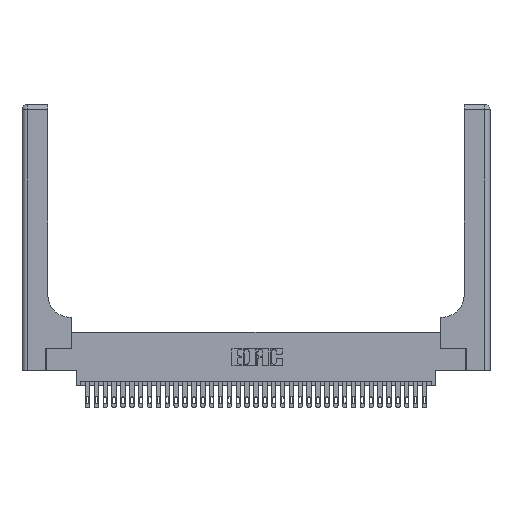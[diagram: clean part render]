
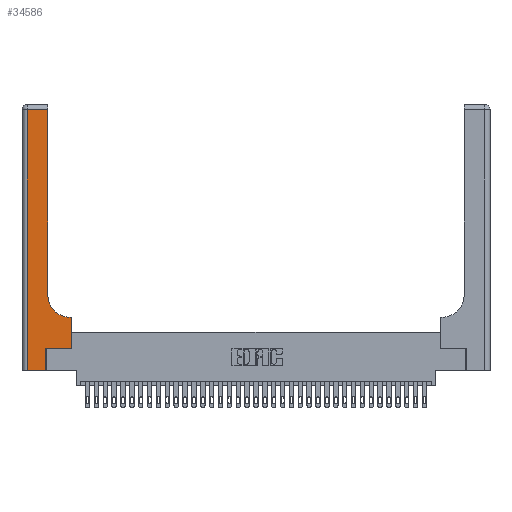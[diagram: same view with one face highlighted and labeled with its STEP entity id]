
A CAD part, top view. The second image highlights one B-rep face of the part: STEP entity #34586.
In plain terms, the highlighted planar face has unit normal (0, 0, 1).
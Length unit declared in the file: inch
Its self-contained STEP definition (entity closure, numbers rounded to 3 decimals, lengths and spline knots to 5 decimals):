
#30 = CARTESIAN_POINT ( 'NONE',  ( 0.2915, 0.85, 0.37 ) ) ;
#225 = DIRECTION ( 'NONE',  ( -1., 0., 0. ) ) ;
#1640 = CARTESIAN_POINT ( 'NONE',  ( 0.269, 0.25, 0.37 ) ) ;
#2290 = CARTESIAN_POINT ( 'NONE',  ( 0.269, 0.25, 0.37 ) ) ;
#2312 = VECTOR ( 'NONE', #16578, 39.37008 ) ;
#2450 = LINE ( 'NONE', #19850, #28628 ) ;
#3448 = PLANE ( 'NONE',  #27595 ) ;
#3651 = ORIENTED_EDGE ( 'NONE', *, *, #24446, .T. ) ;
#3932 = DIRECTION ( 'NONE',  ( 0., 0., -1. ) ) ;
#4219 = VERTEX_POINT ( 'NONE', #20787 ) ;
#4996 = CIRCLE ( 'NONE', #5981, 0.25 ) ;
#5152 = EDGE_CURVE ( 'NONE', #20952, #31302, #27064, .T. ) ;
#5755 = CARTESIAN_POINT ( 'NONE',  ( 0.5585, 0.25, 0.37 ) ) ;
#5981 = AXIS2_PLACEMENT_3D ( 'NONE', #17808, #3932, #23447 ) ;
#6715 = CARTESIAN_POINT ( 'NONE',  ( 0.06, 3., 0.37 ) ) ;
#6752 = VERTEX_POINT ( 'NONE', #28185 ) ;
#7079 = DIRECTION ( 'NONE',  ( 0., -1., 0. ) ) ;
#8183 = EDGE_CURVE ( 'NONE', #4219, #6752, #36016, .T. ) ;
#8776 = DIRECTION ( 'NONE',  ( 1., 0., 0. ) ) ;
#9896 = LINE ( 'NONE', #28507, #20847 ) ;
#11582 = DIRECTION ( 'NONE',  ( 0., 0., -1. ) ) ;
#11962 = VECTOR ( 'NONE', #8776, 39.37008 ) ;
#11964 = VERTEX_POINT ( 'NONE', #20586 ) ;
#12449 = VECTOR ( 'NONE', #34700, 39.37008 ) ;
#13012 = DIRECTION ( 'NONE',  ( 1., 0., 0. ) ) ;
#13886 = DIRECTION ( 'NONE',  ( 0., 1., 0. ) ) ;
#14903 = CARTESIAN_POINT ( 'NONE',  ( 0.2915, 0.6, 0.37 ) ) ;
#15016 = LINE ( 'NONE', #22607, #11962 ) ;
#15380 = CARTESIAN_POINT ( 'NONE',  ( 0.269, 0., 0.37 ) ) ;
#15447 = EDGE_CURVE ( 'NONE', #19894, #4219, #9896, .T. ) ;
#15764 = ORIENTED_EDGE ( 'NONE', *, *, #15447, .T. ) ;
#16008 = EDGE_CURVE ( 'NONE', #33729, #20952, #19485, .T. ) ;
#16038 = CARTESIAN_POINT ( 'NONE',  ( 0.5585, 0.25, 0.37 ) ) ;
#16547 = VECTOR ( 'NONE', #13012, 39.37008 ) ;
#16578 = DIRECTION ( 'NONE',  ( 0., 1., 0. ) ) ;
#17632 = EDGE_CURVE ( 'NONE', #11964, #25515, #33469, .T. ) ;
#17808 = CARTESIAN_POINT ( 'NONE',  ( 0.5415, 0.85, 0.37 ) ) ;
#18071 = EDGE_CURVE ( 'NONE', #25515, #31560, #4996, .T. ) ;
#18116 = ORIENTED_EDGE ( 'NONE', *, *, #18071, .T. ) ;
#18199 = ORIENTED_EDGE ( 'NONE', *, *, #17632, .T. ) ;
#18912 = VECTOR ( 'NONE', #7079, 39.37008 ) ;
#19485 = LINE ( 'NONE', #31962, #12449 ) ;
#19850 = CARTESIAN_POINT ( 'NONE',  ( 0.2915, 3., 0.37 ) ) ;
#19894 = VERTEX_POINT ( 'NONE', #21127 ) ;
#20586 = CARTESIAN_POINT ( 'NONE',  ( 0.5585, 0.6, 0.37 ) ) ;
#20787 = CARTESIAN_POINT ( 'NONE',  ( 0.06, 2.94, 0.37 ) ) ;
#20847 = VECTOR ( 'NONE', #30974, 39.37008 ) ;
#20941 = ORIENTED_EDGE ( 'NONE', *, *, #21779, .T. ) ;
#20952 = VERTEX_POINT ( 'NONE', #2290 ) ;
#21127 = CARTESIAN_POINT ( 'NONE',  ( 0.2915, 2.94, 0.37 ) ) ;
#21779 = EDGE_CURVE ( 'NONE', #31560, #19894, #2450, .T. ) ;
#22607 = CARTESIAN_POINT ( 'NONE',  ( 0., 0., 0.37 ) ) ;
#23447 = DIRECTION ( 'NONE',  ( 1., 0., 0. ) ) ;
#24446 = EDGE_CURVE ( 'NONE', #31302, #11964, #25461, .T. ) ;
#25461 = LINE ( 'NONE', #5755, #2312 ) ;
#25515 = VERTEX_POINT ( 'NONE', #32673 ) ;
#25587 = FACE_OUTER_BOUND ( 'NONE', #32080, .T. ) ;
#25651 = ORIENTED_EDGE ( 'NONE', *, *, #5152, .T. ) ;
#27064 = LINE ( 'NONE', #1640, #16547 ) ;
#27595 = AXIS2_PLACEMENT_3D ( 'NONE', #28339, #11582, #225 ) ;
#28185 = CARTESIAN_POINT ( 'NONE',  ( 0.06, 0., 0.37 ) ) ;
#28339 = CARTESIAN_POINT ( 'NONE',  ( 0., 3., 0.37 ) ) ;
#28507 = CARTESIAN_POINT ( 'NONE',  ( 0., 2.94, 0.37 ) ) ;
#28628 = VECTOR ( 'NONE', #13886, 39.37008 ) ;
#29328 = DIRECTION ( 'NONE',  ( -1., 0., 0. ) ) ;
#30365 = VECTOR ( 'NONE', #29328, 39.37008 ) ;
#30974 = DIRECTION ( 'NONE',  ( -1., 0., 0. ) ) ;
#31054 = ORIENTED_EDGE ( 'NONE', *, *, #16008, .T. ) ;
#31302 = VERTEX_POINT ( 'NONE', #16038 ) ;
#31560 = VERTEX_POINT ( 'NONE', #30 ) ;
#31962 = CARTESIAN_POINT ( 'NONE',  ( 0.269, 0., 0.37 ) ) ;
#32080 = EDGE_LOOP ( 'NONE', ( #20941, #15764, #33858, #34531, #31054, #25651, #3651, #18199, #18116 ) ) ;
#32673 = CARTESIAN_POINT ( 'NONE',  ( 0.5415, 0.6, 0.37 ) ) ;
#33469 = LINE ( 'NONE', #14903, #30365 ) ;
#33729 = VERTEX_POINT ( 'NONE', #15380 ) ;
#33858 = ORIENTED_EDGE ( 'NONE', *, *, #8183, .T. ) ;
#34531 = ORIENTED_EDGE ( 'NONE', *, *, #35194, .T. ) ;
#34586 = ADVANCED_FACE ( 'NONE', ( #25587 ), #3448, .F. ) ;
#34700 = DIRECTION ( 'NONE',  ( 0., 1., 0. ) ) ;
#35194 = EDGE_CURVE ( 'NONE', #6752, #33729, #15016, .T. ) ;
#36016 = LINE ( 'NONE', #6715, #18912 ) ;
